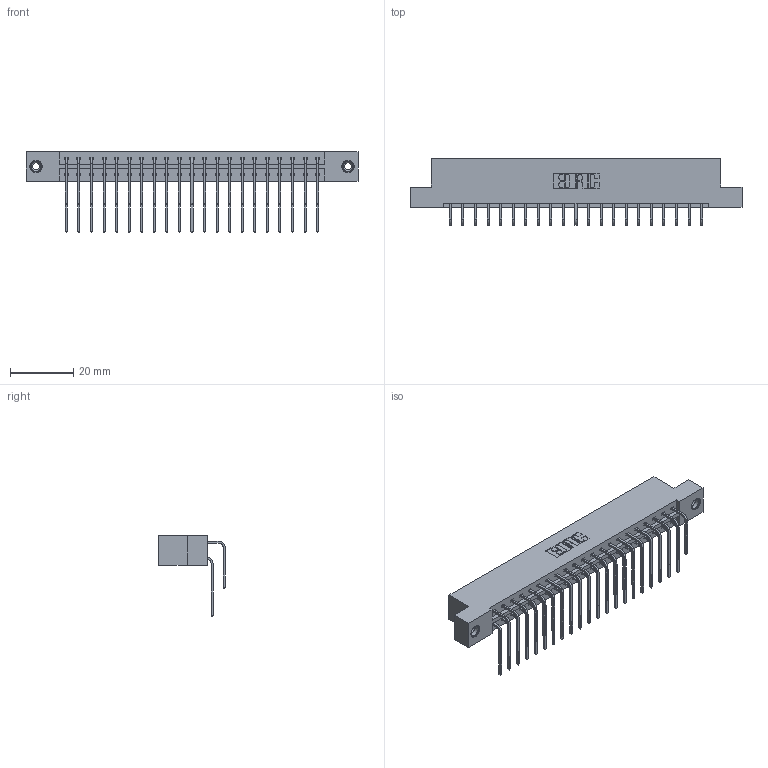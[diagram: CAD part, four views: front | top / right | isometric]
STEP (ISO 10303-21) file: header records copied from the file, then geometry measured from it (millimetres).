
FILE_DESCRIPTION (( 'STEP AP203' ), '1' );
FILE_NAME ('333-042-559-208.STEP', '2018-08-03T19:44:56', ( '' ), ( '' ), 'SwSTEP 2.0', 'SolidWorks 2016', '' );
FILE_SCHEMA (( 'CONFIG_CONTROL_DESIGN' ));
Length unit declared in the file: inch
Products named in the file (5): 333 Part_Flush - .156 Dia - TI; 345-292-001_558 559 Tail - 1; 345-292-001_559 Tail - 2; 345-250-001_345-250-003-102; 333-042-559-208
Assembly tree (45 placements, depth 2):
  333-042-559-208
    333 Part_Flush - .156 Dia - TI
    345-292-001_558 559 Tail - 1  x21
    345-292-001_559 Tail - 2  x21
    345-250-001_345-250-003-102  x2
Bounding box: 104.75 x 20.9 x 25.53 mm (x, y, z)
Volume: 10733.7 mm3; surface area: 13692.9 mm2
Topology: 45 solids, 45 shells, 2442 faces, 7209 edges, 4742 vertices
Faces by surface type: plane 1698, cylinder 728, cone 12, torus 4
Entity records: 19196 total; most frequent: CARTESIAN_POINT 3240, ORIENTED_EDGE 3118, DIRECTION 2817, EDGE_CURVE 1559, VECTOR 1371, LINE 1371, VERTEX_POINT 1032, AXIS2_PLACEMENT_3D 723
